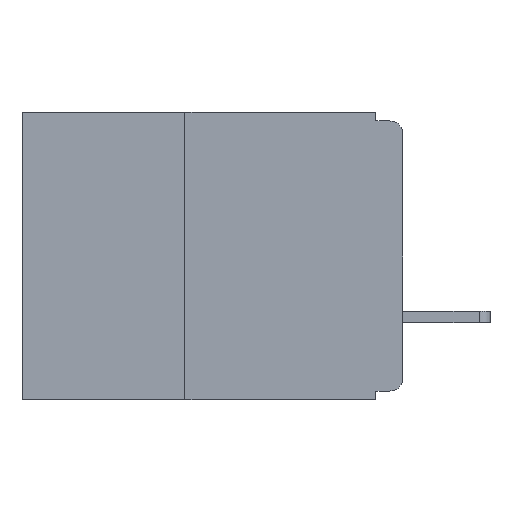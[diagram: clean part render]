
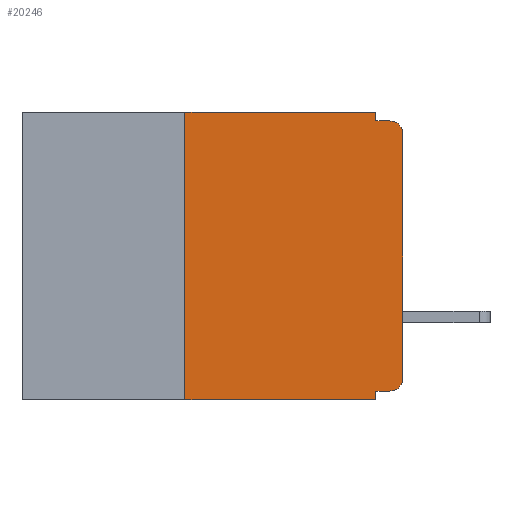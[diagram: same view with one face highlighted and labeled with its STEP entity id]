
A CAD part, left-side view. The second image highlights one B-rep face of the part: STEP entity #20246.
In plain terms, the highlighted planar face has unit normal (-1, 0, 0).
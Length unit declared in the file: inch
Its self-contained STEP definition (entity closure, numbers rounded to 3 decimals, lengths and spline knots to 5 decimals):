
#105 = LINE ( 'NONE', #20088, #15958 ) ;
#263 = LINE ( 'NONE', #11307, #16605 ) ;
#408 = VERTEX_POINT ( 'NONE', #2548 ) ;
#470 = CARTESIAN_POINT ( 'NONE',  ( 0., 0.25, 0. ) ) ;
#670 = VECTOR ( 'NONE', #11124, 39.37008 ) ;
#688 = DIRECTION ( 'NONE',  ( 0., 0., -1. ) ) ;
#1490 = EDGE_CURVE ( 'NONE', #3439, #3260, #16990, .T. ) ;
#1516 = ORIENTED_EDGE ( 'NONE', *, *, #10514, .T. ) ;
#2105 = AXIS2_PLACEMENT_3D ( 'NONE', #4461, #15326, #6053 ) ;
#2321 = VECTOR ( 'NONE', #9528, 39.37008 ) ;
#2418 = LINE ( 'NONE', #10388, #7269 ) ;
#2548 = CARTESIAN_POINT ( 'NONE',  ( 0., 0., -0.305 ) ) ;
#2736 = VERTEX_POINT ( 'NONE', #12574 ) ;
#3026 = FACE_OUTER_BOUND ( 'NONE', #6846, .T. ) ;
#3087 = LINE ( 'NONE', #8329, #15083 ) ;
#3260 = VERTEX_POINT ( 'NONE', #16888 ) ;
#3439 = VERTEX_POINT ( 'NONE', #14181 ) ;
#3545 = CARTESIAN_POINT ( 'NONE',  ( 0., 0., -0.01 ) ) ;
#3621 = DIRECTION ( 'NONE',  ( 0., 0., -1. ) ) ;
#3622 = VERTEX_POINT ( 'NONE', #470 ) ;
#3715 = EDGE_CURVE ( 'NONE', #13993, #3260, #2418, .T. ) ;
#3949 = VECTOR ( 'NONE', #14491, 39.37008 ) ;
#4039 = VERTEX_POINT ( 'NONE', #17177 ) ;
#4158 = EDGE_CURVE ( 'NONE', #19520, #2736, #14940, .T. ) ;
#4294 = DIRECTION ( 'NONE',  ( 1., 0., 0. ) ) ;
#4400 = DIRECTION ( 'NONE',  ( -1., 0., 0. ) ) ;
#4461 = CARTESIAN_POINT ( 'NONE',  ( 0., 0.015, -0.305 ) ) ;
#5567 = LINE ( 'NONE', #8473, #13846 ) ;
#5739 = EDGE_CURVE ( 'NONE', #15616, #13993, #105, .T. ) ;
#6053 = DIRECTION ( 'NONE',  ( 0., 0., -1. ) ) ;
#6623 = ORIENTED_EDGE ( 'NONE', *, *, #10151, .T. ) ;
#6846 = EDGE_LOOP ( 'NONE', ( #6623, #14833, #19355, #11735, #20311, #16762, #13163, #17237, #13636, #1516 ) ) ;
#7245 = CARTESIAN_POINT ( 'NONE',  ( 0., 0.031, -0.32 ) ) ;
#7269 = VECTOR ( 'NONE', #688, 39.37008 ) ;
#7548 = AXIS2_PLACEMENT_3D ( 'NONE', #13642, #4294, #15169 ) ;
#8029 = CARTESIAN_POINT ( 'NONE',  ( 0., 0.437, 0. ) ) ;
#8214 = DIRECTION ( 'NONE',  ( 0., 0., 1. ) ) ;
#8329 = CARTESIAN_POINT ( 'NONE',  ( 0., 0., 0. ) ) ;
#8473 = CARTESIAN_POINT ( 'NONE',  ( 0., 0.031, 0. ) ) ;
#8536 = CARTESIAN_POINT ( 'NONE',  ( 0., 0.015, -0.32 ) ) ;
#9430 = DIRECTION ( 'NONE',  ( 0., 1., 0. ) ) ;
#9528 = DIRECTION ( 'NONE',  ( 0., -1., 0. ) ) ;
#9597 = AXIS2_PLACEMENT_3D ( 'NONE', #13739, #4400, #15269 ) ;
#10108 = CARTESIAN_POINT ( 'NONE',  ( 0., 0.031, -0.01 ) ) ;
#10151 = EDGE_CURVE ( 'NONE', #408, #4039, #3087, .T. ) ;
#10233 = CIRCLE ( 'NONE', #2105, 0.015 ) ;
#10388 = CARTESIAN_POINT ( 'NONE',  ( 0., 0.031, -0.33 ) ) ;
#10514 = EDGE_CURVE ( 'NONE', #15616, #408, #10233, .T. ) ;
#10608 = PLANE ( 'NONE',  #7548 ) ;
#11124 = DIRECTION ( 'NONE',  ( 0., -1., 0. ) ) ;
#11307 = CARTESIAN_POINT ( 'NONE',  ( 0., 0.25, -0.33 ) ) ;
#11735 = ORIENTED_EDGE ( 'NONE', *, *, #15594, .F. ) ;
#12574 = CARTESIAN_POINT ( 'NONE',  ( 0., 0.015, -0.01 ) ) ;
#13163 = ORIENTED_EDGE ( 'NONE', *, *, #1490, .T. ) ;
#13636 = ORIENTED_EDGE ( 'NONE', *, *, #5739, .F. ) ;
#13642 = CARTESIAN_POINT ( 'NONE',  ( 0., 0.437, 0. ) ) ;
#13739 = CARTESIAN_POINT ( 'NONE',  ( 0., 0.015, -0.025 ) ) ;
#13846 = VECTOR ( 'NONE', #3621, 39.37008 ) ;
#13993 = VERTEX_POINT ( 'NONE', #7245 ) ;
#14043 = CARTESIAN_POINT ( 'NONE',  ( 0., 0.437, -0.33 ) ) ;
#14181 = CARTESIAN_POINT ( 'NONE',  ( 0., 0.25, -0.33 ) ) ;
#14277 = VERTEX_POINT ( 'NONE', #18901 ) ;
#14491 = DIRECTION ( 'NONE',  ( 0., -1., 0. ) ) ;
#14833 = ORIENTED_EDGE ( 'NONE', *, *, #15862, .T. ) ;
#14870 = LINE ( 'NONE', #8029, #2321 ) ;
#14940 = LINE ( 'NONE', #3545, #3949 ) ;
#15083 = VECTOR ( 'NONE', #17432, 39.37008 ) ;
#15169 = DIRECTION ( 'NONE',  ( 0., 0., -1. ) ) ;
#15269 = DIRECTION ( 'NONE',  ( 0., 0., -1. ) ) ;
#15326 = DIRECTION ( 'NONE',  ( -1., 0., 0. ) ) ;
#15594 = EDGE_CURVE ( 'NONE', #14277, #19520, #5567, .T. ) ;
#15616 = VERTEX_POINT ( 'NONE', #8536 ) ;
#15862 = EDGE_CURVE ( 'NONE', #4039, #2736, #16713, .T. ) ;
#15958 = VECTOR ( 'NONE', #9430, 39.37008 ) ;
#16605 = VECTOR ( 'NONE', #8214, 39.37008 ) ;
#16713 = CIRCLE ( 'NONE', #9597, 0.015 ) ;
#16762 = ORIENTED_EDGE ( 'NONE', *, *, #17657, .F. ) ;
#16888 = CARTESIAN_POINT ( 'NONE',  ( 0., 0.031, -0.33 ) ) ;
#16990 = LINE ( 'NONE', #14043, #670 ) ;
#17177 = CARTESIAN_POINT ( 'NONE',  ( 0., 0., -0.025 ) ) ;
#17237 = ORIENTED_EDGE ( 'NONE', *, *, #3715, .F. ) ;
#17432 = DIRECTION ( 'NONE',  ( 0., 0., 1. ) ) ;
#17657 = EDGE_CURVE ( 'NONE', #3439, #3622, #263, .T. ) ;
#18817 = EDGE_CURVE ( 'NONE', #3622, #14277, #14870, .T. ) ;
#18901 = CARTESIAN_POINT ( 'NONE',  ( 0., 0.031, 0. ) ) ;
#19355 = ORIENTED_EDGE ( 'NONE', *, *, #4158, .F. ) ;
#19520 = VERTEX_POINT ( 'NONE', #10108 ) ;
#20088 = CARTESIAN_POINT ( 'NONE',  ( 0., 0., -0.32 ) ) ;
#20246 = ADVANCED_FACE ( 'NONE', ( #3026 ), #10608, .F. ) ;
#20311 = ORIENTED_EDGE ( 'NONE', *, *, #18817, .F. ) ;
